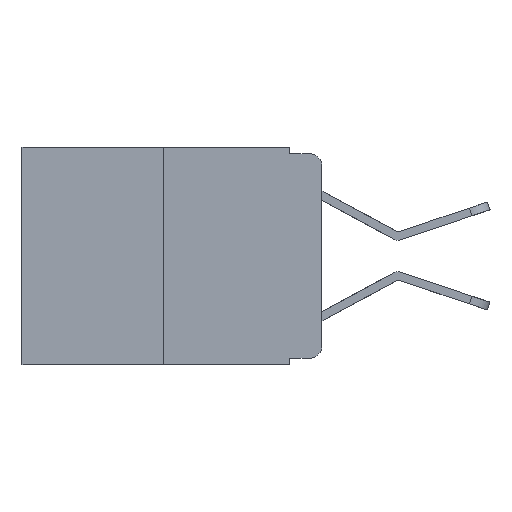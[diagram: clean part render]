
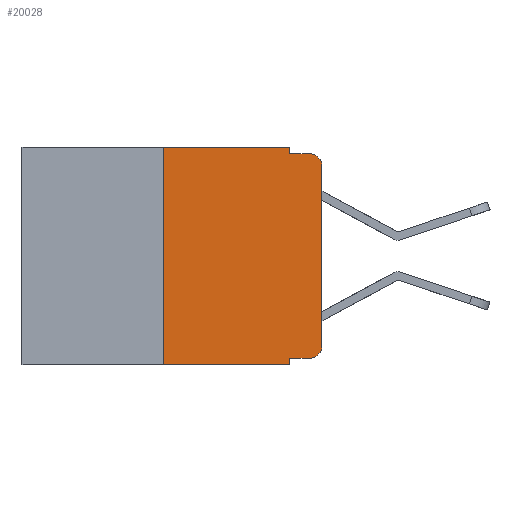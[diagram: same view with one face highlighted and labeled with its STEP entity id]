
A CAD part, left-side view. The second image highlights one B-rep face of the part: STEP entity #20028.
In plain terms, the highlighted planar face has unit normal (-1, 0, 0).
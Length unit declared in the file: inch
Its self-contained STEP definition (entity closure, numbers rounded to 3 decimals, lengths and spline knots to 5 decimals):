
#136 = VECTOR ( 'NONE', #17746, 39.37008 ) ;
#407 = CARTESIAN_POINT ( 'NONE',  ( 0., 0.25, 0. ) ) ;
#431 = VERTEX_POINT ( 'NONE', #18031 ) ;
#489 = ORIENTED_EDGE ( 'NONE', *, *, #12095, .T. ) ;
#496 = DIRECTION ( 'NONE',  ( 0., -1., 0. ) ) ;
#634 = CARTESIAN_POINT ( 'NONE',  ( 0., 0.051, -0.343 ) ) ;
#805 = CARTESIAN_POINT ( 'NONE',  ( 0., 0.051, -0.01 ) ) ;
#1558 = LINE ( 'NONE', #805, #10302 ) ;
#1574 = CARTESIAN_POINT ( 'NONE',  ( 0., 0.051, -0.01 ) ) ;
#1661 = VERTEX_POINT ( 'NONE', #5022 ) ;
#2477 = ORIENTED_EDGE ( 'NONE', *, *, #10697, .F. ) ;
#3045 = ORIENTED_EDGE ( 'NONE', *, *, #8368, .T. ) ;
#4161 = CARTESIAN_POINT ( 'NONE',  ( 0., 0., -0.03 ) ) ;
#4263 = VERTEX_POINT ( 'NONE', #634 ) ;
#4959 = VECTOR ( 'NONE', #10339, 39.37008 ) ;
#5022 = CARTESIAN_POINT ( 'NONE',  ( 0., 0., -0.313 ) ) ;
#5071 = CARTESIAN_POINT ( 'NONE',  ( 0., 0.051, 0. ) ) ;
#5658 = VECTOR ( 'NONE', #5901, 39.37008 ) ;
#5858 = CARTESIAN_POINT ( 'NONE',  ( 0., 0.473, -0.343 ) ) ;
#5880 = EDGE_CURVE ( 'NONE', #9544, #12147, #7079, .T. ) ;
#5901 = DIRECTION ( 'NONE',  ( 0., 0., 1. ) ) ;
#6604 = DIRECTION ( 'NONE',  ( 1., 0., 0. ) ) ;
#7079 = LINE ( 'NONE', #10986, #15592 ) ;
#7145 = EDGE_CURVE ( 'NONE', #12551, #19587, #17643, .T. ) ;
#7258 = AXIS2_PLACEMENT_3D ( 'NONE', #9987, #21740, #11706 ) ;
#7389 = ORIENTED_EDGE ( 'NONE', *, *, #7145, .T. ) ;
#7694 = VECTOR ( 'NONE', #20254, 39.37008 ) ;
#7842 = CARTESIAN_POINT ( 'NONE',  ( 0., 0.02, -0.03 ) ) ;
#8205 = ORIENTED_EDGE ( 'NONE', *, *, #12264, .T. ) ;
#8303 = CARTESIAN_POINT ( 'NONE',  ( 0., 0.051, 0. ) ) ;
#8368 = EDGE_CURVE ( 'NONE', #15254, #4263, #13526, .T. ) ;
#8583 = CARTESIAN_POINT ( 'NONE',  ( 0., 0., 0. ) ) ;
#8673 = CARTESIAN_POINT ( 'NONE',  ( 0., 0.051, -0.333 ) ) ;
#8763 = VERTEX_POINT ( 'NONE', #1574 ) ;
#9536 = ORIENTED_EDGE ( 'NONE', *, *, #9692, .F. ) ;
#9544 = VERTEX_POINT ( 'NONE', #407 ) ;
#9576 = DIRECTION ( 'NONE',  ( 0., 0., -1. ) ) ;
#9692 = EDGE_CURVE ( 'NONE', #8763, #19587, #1558, .T. ) ;
#9987 = CARTESIAN_POINT ( 'NONE',  ( 0., 0.02, -0.313 ) ) ;
#10181 = CARTESIAN_POINT ( 'NONE',  ( 0., 0.051, 0. ) ) ;
#10244 = LINE ( 'NONE', #19383, #5658 ) ;
#10302 = VECTOR ( 'NONE', #14675, 39.37008 ) ;
#10339 = DIRECTION ( 'NONE',  ( 0., 0., 1. ) ) ;
#10697 = EDGE_CURVE ( 'NONE', #15254, #9544, #10244, .T. ) ;
#10798 = CARTESIAN_POINT ( 'NONE',  ( 0., 0.25, -0.343 ) ) ;
#10946 = EDGE_CURVE ( 'NONE', #12147, #8763, #19435, .T. ) ;
#10986 = CARTESIAN_POINT ( 'NONE',  ( 0., 0.473, 0. ) ) ;
#11706 = DIRECTION ( 'NONE',  ( 0., 0., -1. ) ) ;
#12095 = EDGE_CURVE ( 'NONE', #431, #1661, #14667, .T. ) ;
#12113 = FACE_OUTER_BOUND ( 'NONE', #19542, .T. ) ;
#12147 = VERTEX_POINT ( 'NONE', #8303 ) ;
#12264 = EDGE_CURVE ( 'NONE', #15162, #431, #15468, .T. ) ;
#12277 = LINE ( 'NONE', #10181, #7694 ) ;
#12551 = VERTEX_POINT ( 'NONE', #4161 ) ;
#12876 = EDGE_CURVE ( 'NONE', #15162, #4263, #12277, .T. ) ;
#13526 = LINE ( 'NONE', #5858, #136 ) ;
#13721 = CARTESIAN_POINT ( 'NONE',  ( 0., 0.02, -0.01 ) ) ;
#13774 = DIRECTION ( 'NONE',  ( 0., -1., 0. ) ) ;
#14084 = ORIENTED_EDGE ( 'NONE', *, *, #10946, .F. ) ;
#14453 = VECTOR ( 'NONE', #16992, 39.37008 ) ;
#14667 = CIRCLE ( 'NONE', #7258, 0.02 ) ;
#14675 = DIRECTION ( 'NONE',  ( 0., -1., 0. ) ) ;
#14940 = VECTOR ( 'NONE', #13774, 39.37008 ) ;
#15162 = VERTEX_POINT ( 'NONE', #20514 ) ;
#15254 = VERTEX_POINT ( 'NONE', #10798 ) ;
#15468 = LINE ( 'NONE', #8673, #14940 ) ;
#15592 = VECTOR ( 'NONE', #496, 39.37008 ) ;
#15701 = EDGE_CURVE ( 'NONE', #1661, #12551, #18525, .T. ) ;
#16712 = ORIENTED_EDGE ( 'NONE', *, *, #12876, .F. ) ;
#16758 = AXIS2_PLACEMENT_3D ( 'NONE', #16771, #6604, #18458 ) ;
#16771 = CARTESIAN_POINT ( 'NONE',  ( 0., 0.473, 0. ) ) ;
#16992 = DIRECTION ( 'NONE',  ( 0., 0., -1. ) ) ;
#17076 = AXIS2_PLACEMENT_3D ( 'NONE', #7842, #19681, #9576 ) ;
#17643 = CIRCLE ( 'NONE', #17076, 0.02 ) ;
#17746 = DIRECTION ( 'NONE',  ( 0., -1., 0. ) ) ;
#18031 = CARTESIAN_POINT ( 'NONE',  ( 0., 0.02, -0.333 ) ) ;
#18458 = DIRECTION ( 'NONE',  ( 0., 0., -1. ) ) ;
#18525 = LINE ( 'NONE', #8583, #4959 ) ;
#19383 = CARTESIAN_POINT ( 'NONE',  ( 0., 0.25, 0. ) ) ;
#19435 = LINE ( 'NONE', #5071, #14453 ) ;
#19542 = EDGE_LOOP ( 'NONE', ( #20368, #7389, #9536, #14084, #20107, #2477, #3045, #16712, #8205, #489 ) ) ;
#19587 = VERTEX_POINT ( 'NONE', #13721 ) ;
#19681 = DIRECTION ( 'NONE',  ( -1., 0., 0. ) ) ;
#20028 = ADVANCED_FACE ( 'NONE', ( #12113 ), #21736, .F. ) ;
#20107 = ORIENTED_EDGE ( 'NONE', *, *, #5880, .F. ) ;
#20254 = DIRECTION ( 'NONE',  ( 0., 0., -1. ) ) ;
#20368 = ORIENTED_EDGE ( 'NONE', *, *, #15701, .T. ) ;
#20514 = CARTESIAN_POINT ( 'NONE',  ( 0., 0.051, -0.333 ) ) ;
#21736 = PLANE ( 'NONE',  #16758 ) ;
#21740 = DIRECTION ( 'NONE',  ( -1., 0., 0. ) ) ;
